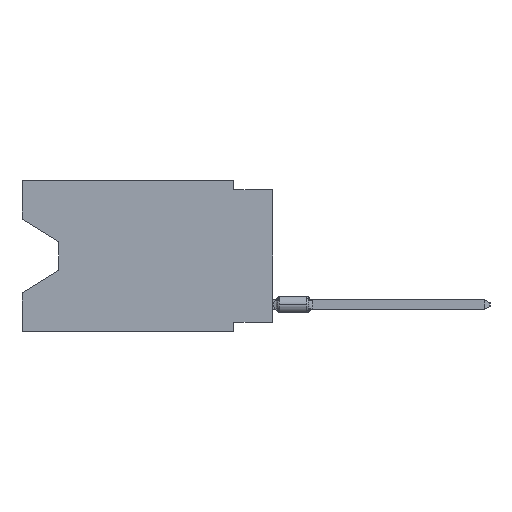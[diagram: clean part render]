
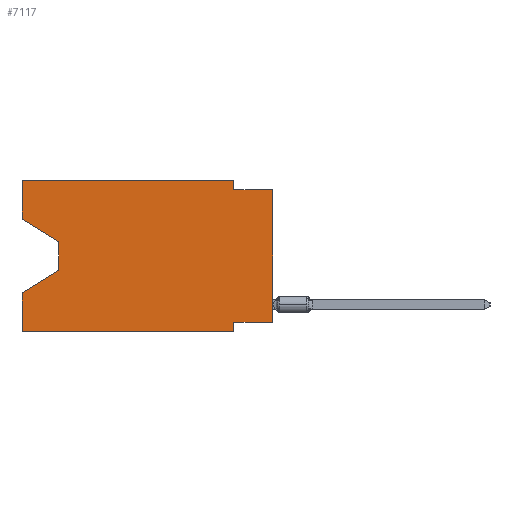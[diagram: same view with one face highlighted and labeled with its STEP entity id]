
A CAD part, left-side view. The second image highlights one B-rep face of the part: STEP entity #7117.
In plain terms, the highlighted planar face has unit normal (-1, 0, 0).
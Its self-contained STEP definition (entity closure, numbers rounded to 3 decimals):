
#2586 = EDGE_CURVE ( 'NONE', #33384, #34769, #37241, .T. ) ;
#2868 = VECTOR ( 'NONE', #59009, 1000. ) ;
#2994 = VERTEX_POINT ( 'NONE', #32624 ) ;
#3384 = EDGE_CURVE ( 'NONE', #12061, #19372, #17133, .T. ) ;
#4365 = LINE ( 'NONE', #61424, #43347 ) ;
#4714 = LINE ( 'NONE', #51507, #31535 ) ;
#6415 = CARTESIAN_POINT ( 'NONE',  ( 0., 2.54, -0.635 ) ) ;
#7117 = ADVANCED_FACE ( 'NONE', ( #19204 ), #40063, .F. ) ;
#7563 = EDGE_CURVE ( 'NONE', #19372, #19722, #44273, .T. ) ;
#8394 = CARTESIAN_POINT ( 'NONE',  ( 0., 2.54, -9.906 ) ) ;
#11194 = LINE ( 'NONE', #17304, #2868 ) ;
#11570 = DIRECTION ( 'NONE',  ( 0., 0.855, -0.519 ) ) ;
#12061 = VERTEX_POINT ( 'NONE', #36220 ) ;
#12446 = EDGE_CURVE ( 'NONE', #47182, #27073, #4365, .T. ) ;
#14083 = CARTESIAN_POINT ( 'NONE',  ( 0., 16.383, 0. ) ) ;
#14597 = DIRECTION ( 'NONE',  ( 0., 0., -1. ) ) ;
#14972 = CARTESIAN_POINT ( 'NONE',  ( 0., 0., -0.635 ) ) ;
#15341 = CARTESIAN_POINT ( 'NONE',  ( 0., 2.54, -9.906 ) ) ;
#16374 = CARTESIAN_POINT ( 'NONE',  ( 0., 2.54, 0. ) ) ;
#17133 = LINE ( 'NONE', #53707, #31737 ) ;
#17304 = CARTESIAN_POINT ( 'NONE',  ( 0., 16.383, -2.546 ) ) ;
#19204 = FACE_OUTER_BOUND ( 'NONE', #43459, .T. ) ;
#19357 = EDGE_CURVE ( 'NONE', #58870, #29366, #42407, .T. ) ;
#19372 = VERTEX_POINT ( 'NONE', #59799 ) ;
#19722 = VERTEX_POINT ( 'NONE', #15341 ) ;
#20067 = DIRECTION ( 'NONE',  ( 0., 0., 1. ) ) ;
#20090 = VECTOR ( 'NONE', #54519, 1000. ) ;
#21818 = CARTESIAN_POINT ( 'NONE',  ( 0., 13.97, -5.893 ) ) ;
#22017 = VECTOR ( 'NONE', #62922, 1000. ) ;
#22312 = EDGE_CURVE ( 'NONE', #29366, #33384, #64770, .T. ) ;
#22346 = VECTOR ( 'NONE', #65590, 1000. ) ;
#22713 = CARTESIAN_POINT ( 'NONE',  ( 0., 13.97, -4.013 ) ) ;
#23750 = VECTOR ( 'NONE', #11570, 1000. ) ;
#24027 = VERTEX_POINT ( 'NONE', #49716 ) ;
#24987 = EDGE_CURVE ( 'NONE', #34769, #2994, #46079, .T. ) ;
#27062 = DIRECTION ( 'NONE',  ( 0., 1., 0. ) ) ;
#27073 = VERTEX_POINT ( 'NONE', #55416 ) ;
#27809 = VECTOR ( 'NONE', #35156, 1000. ) ;
#29366 = VERTEX_POINT ( 'NONE', #50206 ) ;
#29774 = DIRECTION ( 'NONE',  ( 0., -1., 0. ) ) ;
#31535 = VECTOR ( 'NONE', #20067, 1000. ) ;
#31737 = VECTOR ( 'NONE', #27062, 1000. ) ;
#32022 = AXIS2_PLACEMENT_3D ( 'NONE', #14083, #55777, #52662 ) ;
#32181 = CARTESIAN_POINT ( 'NONE',  ( 0., 16.383, -2.546 ) ) ;
#32624 = CARTESIAN_POINT ( 'NONE',  ( 0., 0., -0.635 ) ) ;
#32873 = ORIENTED_EDGE ( 'NONE', *, *, #12446, .T. ) ;
#33129 = ORIENTED_EDGE ( 'NONE', *, *, #55062, .T. ) ;
#33346 = DIRECTION ( 'NONE',  ( 0., -1., 0. ) ) ;
#33384 = VERTEX_POINT ( 'NONE', #44215 ) ;
#33605 = ORIENTED_EDGE ( 'NONE', *, *, #45503, .T. ) ;
#34711 = ORIENTED_EDGE ( 'NONE', *, *, #60357, .F. ) ;
#34769 = VERTEX_POINT ( 'NONE', #6415 ) ;
#35141 = VECTOR ( 'NONE', #29774, 1000. ) ;
#35156 = DIRECTION ( 'NONE',  ( 0., 0., 1. ) ) ;
#35539 = ORIENTED_EDGE ( 'NONE', *, *, #63466, .T. ) ;
#36137 = VERTEX_POINT ( 'NONE', #59775 ) ;
#36220 = CARTESIAN_POINT ( 'NONE',  ( 0., 0., -9.271 ) ) ;
#37241 = LINE ( 'NONE', #16374, #40354 ) ;
#39361 = LINE ( 'NONE', #50948, #35141 ) ;
#40063 = PLANE ( 'NONE',  #32022 ) ;
#40354 = VECTOR ( 'NONE', #58077, 1000. ) ;
#40783 = VECTOR ( 'NONE', #33346, 1000. ) ;
#42071 = CARTESIAN_POINT ( 'NONE',  ( 0., 16.383, 0. ) ) ;
#42323 = ORIENTED_EDGE ( 'NONE', *, *, #2586, .F. ) ;
#42407 = LINE ( 'NONE', #42071, #22017 ) ;
#43347 = VECTOR ( 'NONE', #14597, 1000. ) ;
#43459 = EDGE_LOOP ( 'NONE', ( #33605, #32873, #35539, #34711, #33129, #44266, #63335, #66643, #49197, #42323, #46879, #52930 ) ) ;
#44215 = CARTESIAN_POINT ( 'NONE',  ( 0., 2.54, 0. ) ) ;
#44266 = ORIENTED_EDGE ( 'NONE', *, *, #7563, .F. ) ;
#44273 = LINE ( 'NONE', #8394, #20090 ) ;
#45073 = CARTESIAN_POINT ( 'NONE',  ( 0., 16.383, 0. ) ) ;
#45503 = EDGE_CURVE ( 'NONE', #58870, #47182, #11194, .T. ) ;
#46079 = LINE ( 'NONE', #14972, #22346 ) ;
#46879 = ORIENTED_EDGE ( 'NONE', *, *, #22312, .F. ) ;
#47182 = VERTEX_POINT ( 'NONE', #22713 ) ;
#49197 = ORIENTED_EDGE ( 'NONE', *, *, #24987, .F. ) ;
#49716 = CARTESIAN_POINT ( 'NONE',  ( 0., 16.383, -7.36 ) ) ;
#50206 = CARTESIAN_POINT ( 'NONE',  ( 0., 16.383, 0. ) ) ;
#50948 = CARTESIAN_POINT ( 'NONE',  ( 0., 16.383, -9.906 ) ) ;
#51507 = CARTESIAN_POINT ( 'NONE',  ( 0., 0., 0. ) ) ;
#52662 = DIRECTION ( 'NONE',  ( 0., 0., -1. ) ) ;
#52930 = ORIENTED_EDGE ( 'NONE', *, *, #19357, .F. ) ;
#53251 = LINE ( 'NONE', #21818, #23750 ) ;
#53707 = CARTESIAN_POINT ( 'NONE',  ( 0., 0., -9.271 ) ) ;
#54519 = DIRECTION ( 'NONE',  ( 0., 0., -1. ) ) ;
#55062 = EDGE_CURVE ( 'NONE', #36137, #19722, #39361, .T. ) ;
#55416 = CARTESIAN_POINT ( 'NONE',  ( 0., 13.97, -5.893 ) ) ;
#55777 = DIRECTION ( 'NONE',  ( 1., 0., 0. ) ) ;
#58077 = DIRECTION ( 'NONE',  ( 0., 0., -1. ) ) ;
#58870 = VERTEX_POINT ( 'NONE', #32181 ) ;
#59009 = DIRECTION ( 'NONE',  ( 0., -0.855, -0.519 ) ) ;
#59296 = CARTESIAN_POINT ( 'NONE',  ( 0., 16.383, 0. ) ) ;
#59775 = CARTESIAN_POINT ( 'NONE',  ( 0., 16.383, -9.906 ) ) ;
#59799 = CARTESIAN_POINT ( 'NONE',  ( 0., 2.54, -9.271 ) ) ;
#60357 = EDGE_CURVE ( 'NONE', #36137, #24027, #61799, .T. ) ;
#61424 = CARTESIAN_POINT ( 'NONE',  ( 0., 13.97, -4.013 ) ) ;
#61799 = LINE ( 'NONE', #45073, #27809 ) ;
#62922 = DIRECTION ( 'NONE',  ( 0., 0., 1. ) ) ;
#63335 = ORIENTED_EDGE ( 'NONE', *, *, #3384, .F. ) ;
#63466 = EDGE_CURVE ( 'NONE', #27073, #24027, #53251, .T. ) ;
#64770 = LINE ( 'NONE', #59296, #40783 ) ;
#65219 = EDGE_CURVE ( 'NONE', #12061, #2994, #4714, .T. ) ;
#65590 = DIRECTION ( 'NONE',  ( 0., -1., 0. ) ) ;
#66643 = ORIENTED_EDGE ( 'NONE', *, *, #65219, .T. ) ;
